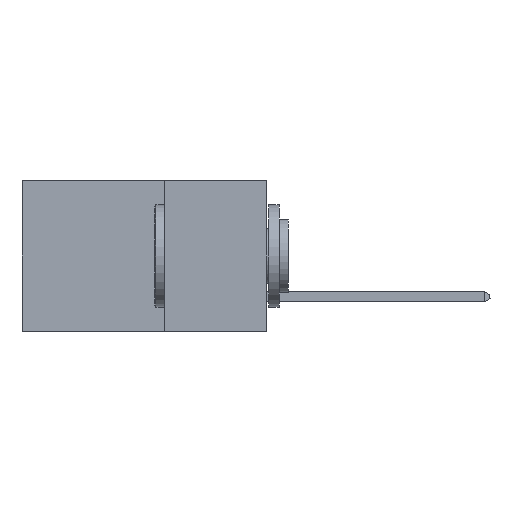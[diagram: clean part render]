
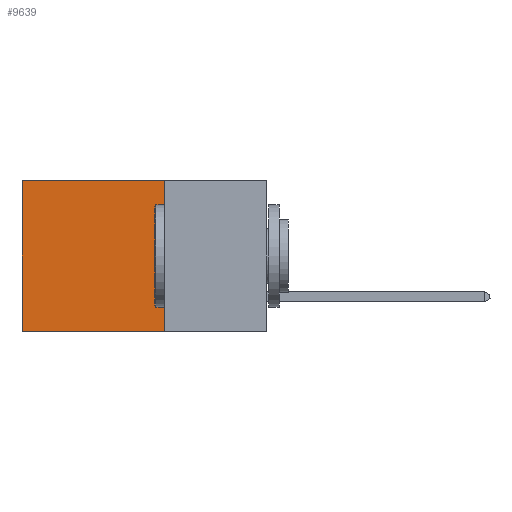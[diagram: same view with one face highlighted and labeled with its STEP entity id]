
A CAD part, left-side view. The second image highlights one B-rep face of the part: STEP entity #9639.
In plain terms, the highlighted planar face has unit normal (-1, 0, 0).
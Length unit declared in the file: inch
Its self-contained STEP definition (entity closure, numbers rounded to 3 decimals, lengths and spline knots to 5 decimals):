
#2668 = EDGE_LOOP ( 'NONE', ( #20084, #10733, #23866, #33603 ) ) ;
#3012 = DIRECTION ( 'NONE',  ( 0., 0., -1. ) ) ;
#4929 = VECTOR ( 'NONE', #10494, 39.37008 ) ;
#5486 = FACE_OUTER_BOUND ( 'NONE', #2668, .T. ) ;
#5682 = CARTESIAN_POINT ( 'NONE',  ( 0.2875, 0.25, 0. ) ) ;
#6920 = DIRECTION ( 'NONE',  ( 0., 1., 0. ) ) ;
#7110 = DIRECTION ( 'NONE',  ( 0., 1., 0. ) ) ;
#7341 = CARTESIAN_POINT ( 'NONE',  ( 0.2875, 0.25, 0. ) ) ;
#8156 = VECTOR ( 'NONE', #6920, 39.37008 ) ;
#8720 = PLANE ( 'NONE',  #15872 ) ;
#8858 = DIRECTION ( 'NONE',  ( 1., 0., 0. ) ) ;
#9639 = ADVANCED_FACE ( 'NONE', ( #5486 ), #8720, .F. ) ;
#10494 = DIRECTION ( 'NONE',  ( 0., 0., -1. ) ) ;
#10733 = ORIENTED_EDGE ( 'NONE', *, *, #33116, .F. ) ;
#11649 = CARTESIAN_POINT ( 'NONE',  ( 0.2875, 0.25, -0.37 ) ) ;
#15214 = LINE ( 'NONE', #7341, #4929 ) ;
#15480 = LINE ( 'NONE', #21716, #31954 ) ;
#15734 = VERTEX_POINT ( 'NONE', #11649 ) ;
#15872 = AXIS2_PLACEMENT_3D ( 'NONE', #5682, #8858, #30547 ) ;
#16402 = LINE ( 'NONE', #34583, #8156 ) ;
#16772 = EDGE_CURVE ( 'NONE', #32162, #15734, #15214, .T. ) ;
#17194 = EDGE_CURVE ( 'NONE', #32162, #40259, #32631, .T. ) ;
#20084 = ORIENTED_EDGE ( 'NONE', *, *, #35845, .T. ) ;
#21716 = CARTESIAN_POINT ( 'NONE',  ( 0.2875, 0.6, 0. ) ) ;
#22720 = CARTESIAN_POINT ( 'NONE',  ( 0.2875, 0.25, 0. ) ) ;
#23866 = ORIENTED_EDGE ( 'NONE', *, *, #16772, .F. ) ;
#24449 = VERTEX_POINT ( 'NONE', #34455 ) ;
#24494 = CARTESIAN_POINT ( 'NONE',  ( 0.2875, 0.6, 0. ) ) ;
#29638 = CARTESIAN_POINT ( 'NONE',  ( 0.2875, 0.25, 0. ) ) ;
#30547 = DIRECTION ( 'NONE',  ( 0., 0., -1. ) ) ;
#31954 = VECTOR ( 'NONE', #3012, 39.37008 ) ;
#32162 = VERTEX_POINT ( 'NONE', #29638 ) ;
#32631 = LINE ( 'NONE', #22720, #39843 ) ;
#33116 = EDGE_CURVE ( 'NONE', #15734, #24449, #16402, .T. ) ;
#33603 = ORIENTED_EDGE ( 'NONE', *, *, #17194, .T. ) ;
#34455 = CARTESIAN_POINT ( 'NONE',  ( 0.2875, 0.6, -0.37 ) ) ;
#34583 = CARTESIAN_POINT ( 'NONE',  ( 0.2875, 0.25, -0.37 ) ) ;
#35845 = EDGE_CURVE ( 'NONE', #40259, #24449, #15480, .T. ) ;
#39843 = VECTOR ( 'NONE', #7110, 39.37008 ) ;
#40259 = VERTEX_POINT ( 'NONE', #24494 ) ;
